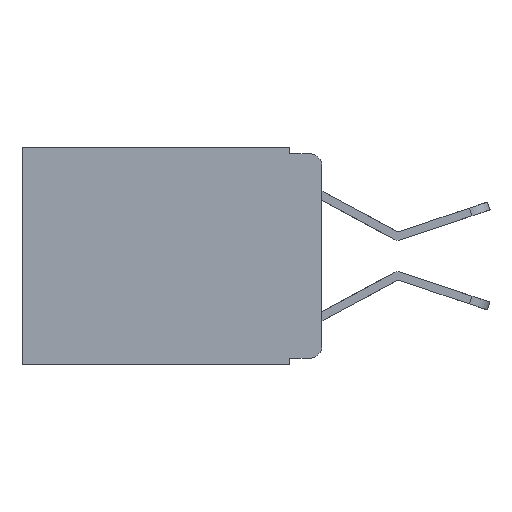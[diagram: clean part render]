
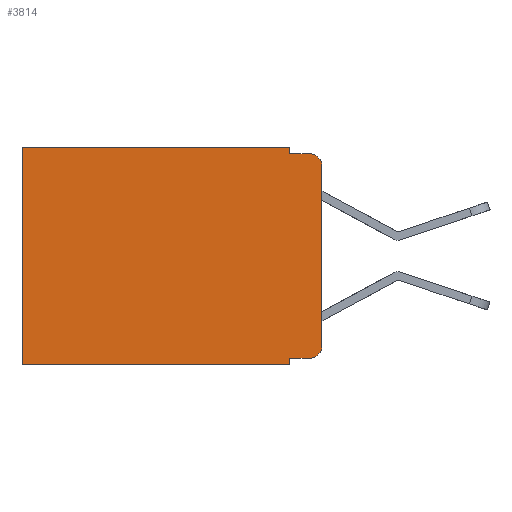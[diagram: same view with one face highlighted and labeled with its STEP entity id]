
A CAD part, left-side view. The second image highlights one B-rep face of the part: STEP entity #3814.
In plain terms, the highlighted planar face has unit normal (-1, 0, 0).
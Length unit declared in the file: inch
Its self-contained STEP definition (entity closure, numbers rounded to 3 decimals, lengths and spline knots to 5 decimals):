
#156 = CARTESIAN_POINT ( 'NONE',  ( 0.298, 0.02, -0.313 ) ) ;
#253 = VERTEX_POINT ( 'NONE', #10557 ) ;
#264 = CIRCLE ( 'NONE', #4987, 0.02 ) ;
#276 = CARTESIAN_POINT ( 'NONE',  ( 0.298, 0.02, -0.03 ) ) ;
#328 = DIRECTION ( 'NONE',  ( 0., 0., -1. ) ) ;
#354 = VERTEX_POINT ( 'NONE', #9567 ) ;
#408 = EDGE_CURVE ( 'NONE', #9811, #9910, #2013, .T. ) ;
#439 = ORIENTED_EDGE ( 'NONE', *, *, #9189, .F. ) ;
#554 = ORIENTED_EDGE ( 'NONE', *, *, #10449, .T. ) ;
#691 = EDGE_CURVE ( 'NONE', #6885, #5847, #8420, .T. ) ;
#1011 = DIRECTION ( 'NONE',  ( 0., 0., -1. ) ) ;
#1022 = DIRECTION ( 'NONE',  ( 0., 0., -1. ) ) ;
#1128 = LINE ( 'NONE', #7144, #10390 ) ;
#1140 = CARTESIAN_POINT ( 'NONE',  ( 0.298, 0.02, -0.01 ) ) ;
#1199 = CARTESIAN_POINT ( 'NONE',  ( 0.298, 0.051, 0. ) ) ;
#1283 = CIRCLE ( 'NONE', #7932, 0.02 ) ;
#1295 = VECTOR ( 'NONE', #1011, 39.37008 ) ;
#1521 = CARTESIAN_POINT ( 'NONE',  ( 0.298, 0., 0. ) ) ;
#1577 = DIRECTION ( 'NONE',  ( -1., 0., 0. ) ) ;
#1796 = DIRECTION ( 'NONE',  ( 0., 0., -1. ) ) ;
#1881 = LINE ( 'NONE', #10157, #1295 ) ;
#1905 = ORIENTED_EDGE ( 'NONE', *, *, #7666, .T. ) ;
#2013 = LINE ( 'NONE', #3766, #7504 ) ;
#2253 = CARTESIAN_POINT ( 'NONE',  ( 0.298, 0.051, -0.01 ) ) ;
#2853 = DIRECTION ( 'NONE',  ( -1., 0., 0. ) ) ;
#2919 = ORIENTED_EDGE ( 'NONE', *, *, #408, .F. ) ;
#3515 = DIRECTION ( 'NONE',  ( 1., 0., 0. ) ) ;
#3719 = AXIS2_PLACEMENT_3D ( 'NONE', #9859, #3515, #1796 ) ;
#3766 = CARTESIAN_POINT ( 'NONE',  ( 0.298, 0., 0. ) ) ;
#3789 = EDGE_LOOP ( 'NONE', ( #2919, #5226, #10423, #9558, #554, #9553, #3806, #439, #1905, #7247 ) ) ;
#3806 = ORIENTED_EDGE ( 'NONE', *, *, #8223, .F. ) ;
#3814 = ADVANCED_FACE ( 'NONE', ( #5651 ), #8984, .F. ) ;
#3865 = DIRECTION ( 'NONE',  ( 0., 1., 0. ) ) ;
#4214 = VERTEX_POINT ( 'NONE', #9624 ) ;
#4475 = DIRECTION ( 'NONE',  ( 0., -1., 0. ) ) ;
#4685 = LINE ( 'NONE', #9873, #9184 ) ;
#4987 = AXIS2_PLACEMENT_3D ( 'NONE', #276, #2853, #328 ) ;
#5015 = VERTEX_POINT ( 'NONE', #9808 ) ;
#5182 = EDGE_CURVE ( 'NONE', #6482, #253, #8536, .T. ) ;
#5226 = ORIENTED_EDGE ( 'NONE', *, *, #9573, .T. ) ;
#5651 = FACE_OUTER_BOUND ( 'NONE', #3789, .T. ) ;
#5675 = VECTOR ( 'NONE', #5867, 39.37008 ) ;
#5738 = DIRECTION ( 'NONE',  ( 0., 0., -1. ) ) ;
#5847 = VERTEX_POINT ( 'NONE', #1140 ) ;
#5867 = DIRECTION ( 'NONE',  ( 0., -1., 0. ) ) ;
#6014 = EDGE_CURVE ( 'NONE', #9654, #6885, #8198, .T. ) ;
#6482 = VERTEX_POINT ( 'NONE', #10480 ) ;
#6885 = VERTEX_POINT ( 'NONE', #2253 ) ;
#7096 = DIRECTION ( 'NONE',  ( 0., 0., -1. ) ) ;
#7144 = CARTESIAN_POINT ( 'NONE',  ( 0.298, 0.051, -0.333 ) ) ;
#7247 = ORIENTED_EDGE ( 'NONE', *, *, #8839, .T. ) ;
#7489 = DIRECTION ( 'NONE',  ( 0., 1., 0. ) ) ;
#7497 = CARTESIAN_POINT ( 'NONE',  ( 0.298, 0.051, -0.01 ) ) ;
#7504 = VECTOR ( 'NONE', #7096, 39.37008 ) ;
#7656 = DIRECTION ( 'NONE',  ( 0., 0., -1. ) ) ;
#7666 = EDGE_CURVE ( 'NONE', #354, #4214, #1128, .T. ) ;
#7932 = AXIS2_PLACEMENT_3D ( 'NONE', #156, #1577, #1022 ) ;
#8109 = CARTESIAN_POINT ( 'NONE',  ( 0.298, 0., -0.313 ) ) ;
#8198 = LINE ( 'NONE', #8960, #10707 ) ;
#8223 = EDGE_CURVE ( 'NONE', #5015, #253, #4685, .T. ) ;
#8376 = CARTESIAN_POINT ( 'NONE',  ( 0.298, 0.473, 0. ) ) ;
#8420 = LINE ( 'NONE', #7497, #5675 ) ;
#8536 = LINE ( 'NONE', #8376, #10700 ) ;
#8550 = CARTESIAN_POINT ( 'NONE',  ( 0.298, 0., -0.03 ) ) ;
#8839 = EDGE_CURVE ( 'NONE', #4214, #9910, #1283, .T. ) ;
#8849 = VECTOR ( 'NONE', #7489, 39.37008 ) ;
#8960 = CARTESIAN_POINT ( 'NONE',  ( 0.298, 0.051, 0. ) ) ;
#8984 = PLANE ( 'NONE',  #3719 ) ;
#9184 = VECTOR ( 'NONE', #3865, 39.37008 ) ;
#9189 = EDGE_CURVE ( 'NONE', #354, #5015, #1881, .T. ) ;
#9553 = ORIENTED_EDGE ( 'NONE', *, *, #5182, .T. ) ;
#9558 = ORIENTED_EDGE ( 'NONE', *, *, #6014, .F. ) ;
#9567 = CARTESIAN_POINT ( 'NONE',  ( 0.298, 0.051, -0.333 ) ) ;
#9573 = EDGE_CURVE ( 'NONE', #9811, #5847, #264, .T. ) ;
#9624 = CARTESIAN_POINT ( 'NONE',  ( 0.298, 0.02, -0.333 ) ) ;
#9654 = VERTEX_POINT ( 'NONE', #1199 ) ;
#9808 = CARTESIAN_POINT ( 'NONE',  ( 0.298, 0.051, -0.343 ) ) ;
#9811 = VERTEX_POINT ( 'NONE', #8550 ) ;
#9859 = CARTESIAN_POINT ( 'NONE',  ( 0.298, 0., 0. ) ) ;
#9873 = CARTESIAN_POINT ( 'NONE',  ( 0.298, 0., -0.343 ) ) ;
#9910 = VERTEX_POINT ( 'NONE', #8109 ) ;
#10157 = CARTESIAN_POINT ( 'NONE',  ( 0.298, 0.051, 0. ) ) ;
#10390 = VECTOR ( 'NONE', #4475, 39.37008 ) ;
#10423 = ORIENTED_EDGE ( 'NONE', *, *, #691, .F. ) ;
#10449 = EDGE_CURVE ( 'NONE', #9654, #6482, #10664, .T. ) ;
#10480 = CARTESIAN_POINT ( 'NONE',  ( 0.298, 0.473, 0. ) ) ;
#10557 = CARTESIAN_POINT ( 'NONE',  ( 0.298, 0.473, -0.343 ) ) ;
#10664 = LINE ( 'NONE', #1521, #8849 ) ;
#10700 = VECTOR ( 'NONE', #7656, 39.37008 ) ;
#10707 = VECTOR ( 'NONE', #5738, 39.37008 ) ;
